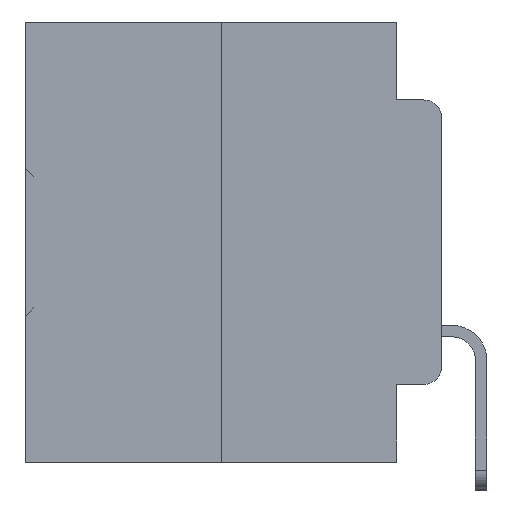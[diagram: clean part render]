
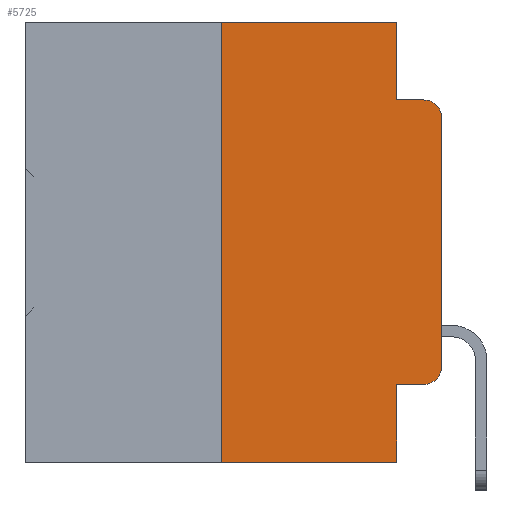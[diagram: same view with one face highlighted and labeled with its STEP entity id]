
A CAD part, left-side view. The second image highlights one B-rep face of the part: STEP entity #5725.
In plain terms, the highlighted planar face has unit normal (-1, 0, 0).
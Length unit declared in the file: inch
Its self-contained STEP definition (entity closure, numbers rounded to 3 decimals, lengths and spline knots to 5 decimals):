
#317 = VERTEX_POINT ( 'NONE', #13238 ) ;
#377 = VECTOR ( 'NONE', #28753, 39.37008 ) ;
#1029 = LINE ( 'NONE', #13112, #8040 ) ;
#1434 = VERTEX_POINT ( 'NONE', #18293 ) ;
#2452 = CARTESIAN_POINT ( 'NONE',  ( 0., 0.051, 0. ) ) ;
#3162 = CARTESIAN_POINT ( 'NONE',  ( 0., 0.25, 0. ) ) ;
#3612 = CARTESIAN_POINT ( 'NONE',  ( 0., 0.473, 0. ) ) ;
#3859 = CARTESIAN_POINT ( 'NONE',  ( 0., 0., 0. ) ) ;
#4466 = VERTEX_POINT ( 'NONE', #32765 ) ;
#4816 = EDGE_LOOP ( 'NONE', ( #23594, #9834, #19501, #36699, #7589, #25886, #20875, #8080, #16780, #10806 ) ) ;
#5725 = ADVANCED_FACE ( 'NONE', ( #14986 ), #17400, .F. ) ;
#6711 = DIRECTION ( 'NONE',  ( 0., -1., 0. ) ) ;
#7589 = ORIENTED_EDGE ( 'NONE', *, *, #27904, .F. ) ;
#8040 = VECTOR ( 'NONE', #36360, 39.37008 ) ;
#8080 = ORIENTED_EDGE ( 'NONE', *, *, #12129, .F. ) ;
#8323 = LINE ( 'NONE', #22797, #377 ) ;
#9422 = EDGE_CURVE ( 'NONE', #13281, #4466, #31202, .T. ) ;
#9748 = CARTESIAN_POINT ( 'NONE',  ( 0., 0.02, -0.4115 ) ) ;
#9828 = LINE ( 'NONE', #3859, #16736 ) ;
#9834 = ORIENTED_EDGE ( 'NONE', *, *, #9422, .T. ) ;
#10158 = EDGE_CURVE ( 'NONE', #15462, #34353, #20768, .T. ) ;
#10637 = CARTESIAN_POINT ( 'NONE',  ( 0., 0.25, 0. ) ) ;
#10806 = ORIENTED_EDGE ( 'NONE', *, *, #36226, .T. ) ;
#11942 = LINE ( 'NONE', #3612, #34242 ) ;
#12129 = EDGE_CURVE ( 'NONE', #15462, #317, #36456, .T. ) ;
#12150 = DIRECTION ( 'NONE',  ( -1., 0., 0. ) ) ;
#13112 = CARTESIAN_POINT ( 'NONE',  ( 0., 0.051, 0. ) ) ;
#13238 = CARTESIAN_POINT ( 'NONE',  ( 0., 0.051, -0.5 ) ) ;
#13281 = VERTEX_POINT ( 'NONE', #28145 ) ;
#14259 = CARTESIAN_POINT ( 'NONE',  ( 0., 0.051, -0.4115 ) ) ;
#14443 = CARTESIAN_POINT ( 'NONE',  ( 0., 0.473, 0. ) ) ;
#14689 = DIRECTION ( 'NONE',  ( -1., 0., 0. ) ) ;
#14986 = FACE_OUTER_BOUND ( 'NONE', #4816, .T. ) ;
#15462 = VERTEX_POINT ( 'NONE', #14259 ) ;
#15913 = VECTOR ( 'NONE', #19488, 39.37008 ) ;
#16736 = VECTOR ( 'NONE', #27339, 39.37008 ) ;
#16780 = ORIENTED_EDGE ( 'NONE', *, *, #10158, .T. ) ;
#17139 = AXIS2_PLACEMENT_3D ( 'NONE', #14443, #23136, #20333 ) ;
#17400 = PLANE ( 'NONE',  #17139 ) ;
#17471 = AXIS2_PLACEMENT_3D ( 'NONE', #29629, #12150, #32510 ) ;
#18293 = CARTESIAN_POINT ( 'NONE',  ( 0., 0., -0.3915 ) ) ;
#19488 = DIRECTION ( 'NONE',  ( 0., 0., 1. ) ) ;
#19501 = ORIENTED_EDGE ( 'NONE', *, *, #35521, .F. ) ;
#20333 = DIRECTION ( 'NONE',  ( 0., 0., -1. ) ) ;
#20768 = LINE ( 'NONE', #32954, #27599 ) ;
#20854 = CARTESIAN_POINT ( 'NONE',  ( 0., 0.051, 0. ) ) ;
#20875 = ORIENTED_EDGE ( 'NONE', *, *, #35575, .T. ) ;
#21963 = EDGE_CURVE ( 'NONE', #25930, #32264, #24595, .T. ) ;
#22041 = VECTOR ( 'NONE', #37567, 39.37008 ) ;
#22264 = VERTEX_POINT ( 'NONE', #20854 ) ;
#22797 = CARTESIAN_POINT ( 'NONE',  ( 0., 0.051, -0.0885 ) ) ;
#23136 = DIRECTION ( 'NONE',  ( 1., 0., 0. ) ) ;
#23188 = EDGE_CURVE ( 'NONE', #1434, #13281, #9828, .T. ) ;
#23489 = CARTESIAN_POINT ( 'NONE',  ( 0., 0.25, -0.5 ) ) ;
#23594 = ORIENTED_EDGE ( 'NONE', *, *, #23188, .T. ) ;
#23912 = EDGE_CURVE ( 'NONE', #22264, #26260, #1029, .T. ) ;
#24595 = LINE ( 'NONE', #10637, #15913 ) ;
#25886 = ORIENTED_EDGE ( 'NONE', *, *, #21963, .F. ) ;
#25930 = VERTEX_POINT ( 'NONE', #23489 ) ;
#25950 = DIRECTION ( 'NONE',  ( 0., 0., -1. ) ) ;
#26260 = VERTEX_POINT ( 'NONE', #27894 ) ;
#27339 = DIRECTION ( 'NONE',  ( 0., 0., 1. ) ) ;
#27599 = VECTOR ( 'NONE', #6711, 39.37008 ) ;
#27894 = CARTESIAN_POINT ( 'NONE',  ( 0., 0.051, -0.0885 ) ) ;
#27904 = EDGE_CURVE ( 'NONE', #32264, #22264, #11942, .T. ) ;
#28145 = CARTESIAN_POINT ( 'NONE',  ( 0., 0., -0.1085 ) ) ;
#28753 = DIRECTION ( 'NONE',  ( 0., -1., 0. ) ) ;
#29629 = CARTESIAN_POINT ( 'NONE',  ( 0., 0.02, -0.1085 ) ) ;
#29866 = DIRECTION ( 'NONE',  ( 0., -1., 0. ) ) ;
#31202 = CIRCLE ( 'NONE', #17471, 0.02 ) ;
#31769 = CARTESIAN_POINT ( 'NONE',  ( 0., 0.473, -0.5 ) ) ;
#32088 = CARTESIAN_POINT ( 'NONE',  ( 0., 0.02, -0.3915 ) ) ;
#32264 = VERTEX_POINT ( 'NONE', #3162 ) ;
#32510 = DIRECTION ( 'NONE',  ( 0., 0., -1. ) ) ;
#32765 = CARTESIAN_POINT ( 'NONE',  ( 0., 0.02, -0.0885 ) ) ;
#32954 = CARTESIAN_POINT ( 'NONE',  ( 0., 0.051, -0.4115 ) ) ;
#34187 = CIRCLE ( 'NONE', #36704, 0.02 ) ;
#34242 = VECTOR ( 'NONE', #29866, 39.37008 ) ;
#34353 = VERTEX_POINT ( 'NONE', #9748 ) ;
#34995 = DIRECTION ( 'NONE',  ( 0., 0., -1. ) ) ;
#35521 = EDGE_CURVE ( 'NONE', #26260, #4466, #8323, .T. ) ;
#35561 = VECTOR ( 'NONE', #25950, 39.37008 ) ;
#35575 = EDGE_CURVE ( 'NONE', #25930, #317, #37420, .T. ) ;
#36226 = EDGE_CURVE ( 'NONE', #34353, #1434, #34187, .T. ) ;
#36360 = DIRECTION ( 'NONE',  ( 0., 0., -1. ) ) ;
#36456 = LINE ( 'NONE', #2452, #35561 ) ;
#36699 = ORIENTED_EDGE ( 'NONE', *, *, #23912, .F. ) ;
#36704 = AXIS2_PLACEMENT_3D ( 'NONE', #32088, #14689, #34995 ) ;
#37420 = LINE ( 'NONE', #31769, #22041 ) ;
#37567 = DIRECTION ( 'NONE',  ( 0., -1., 0. ) ) ;
